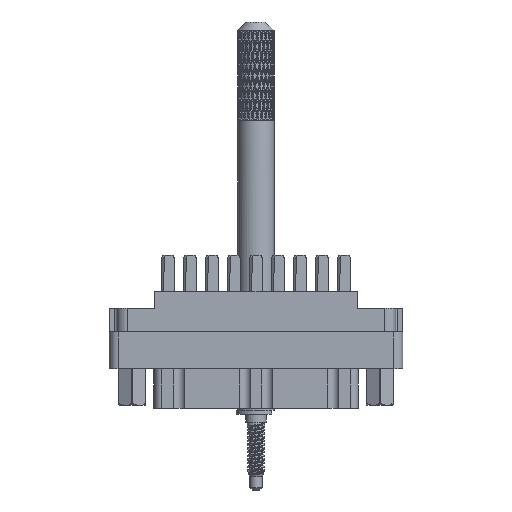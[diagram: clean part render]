
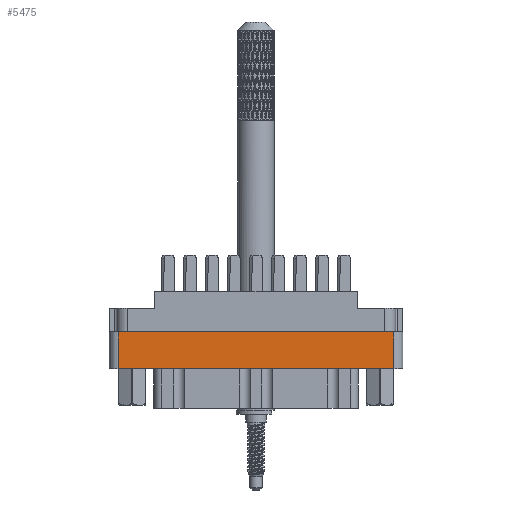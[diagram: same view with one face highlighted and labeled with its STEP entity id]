
A CAD part, front view. The second image highlights one B-rep face of the part: STEP entity #5475.
In plain terms, the highlighted planar face has unit normal (0, -1, 0).
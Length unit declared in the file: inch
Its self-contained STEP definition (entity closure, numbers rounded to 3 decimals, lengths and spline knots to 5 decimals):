
#3279 = PLANE ( 'NONE',  #110647 ) ;
#3313 = VERTEX_POINT ( 'NONE', #109894 ) ;
#5475 = ADVANCED_FACE ( 'NONE', ( #19551 ), #3279, .T. ) ;
#8591 = VECTOR ( 'NONE', #20336, 39.37008 ) ;
#11856 = LINE ( 'NONE', #29251, #79768 ) ;
#14484 = ORIENTED_EDGE ( 'NONE', *, *, #26100, .F. ) ;
#18546 = EDGE_CURVE ( 'NONE', #88867, #25865, #80310, .T. ) ;
#18998 = DIRECTION ( 'NONE',  ( 0., -1., 0. ) ) ;
#19551 = FACE_OUTER_BOUND ( 'NONE', #27443, .T. ) ;
#20336 = DIRECTION ( 'NONE',  ( 0., 0., 1. ) ) ;
#25865 = VERTEX_POINT ( 'NONE', #39438 ) ;
#26100 = EDGE_CURVE ( 'NONE', #36804, #3313, #11856, .T. ) ;
#27443 = EDGE_LOOP ( 'NONE', ( #14484, #83085, #93789, #32451 ) ) ;
#29251 = CARTESIAN_POINT ( 'NONE',  ( -0.938, -0.438, -0.798 ) ) ;
#32451 = ORIENTED_EDGE ( 'NONE', *, *, #77188, .F. ) ;
#36804 = VERTEX_POINT ( 'NONE', #90131 ) ;
#37460 = DIRECTION ( 'NONE',  ( 0., 0., -1. ) ) ;
#39438 = CARTESIAN_POINT ( 'NONE',  ( 0.938, -0.438, -0.277 ) ) ;
#44730 = VECTOR ( 'NONE', #45438, 39.37008 ) ;
#45438 = DIRECTION ( 'NONE',  ( -1., 0., 0. ) ) ;
#54375 = LINE ( 'NONE', #96449, #44730 ) ;
#55544 = EDGE_CURVE ( 'NONE', #88867, #36804, #54375, .T. ) ;
#57271 = DIRECTION ( 'NONE',  ( 1., 0., 0. ) ) ;
#77188 = EDGE_CURVE ( 'NONE', #3313, #25865, #108332, .T. ) ;
#79768 = VECTOR ( 'NONE', #105474, 39.37008 ) ;
#80310 = LINE ( 'NONE', #90946, #8591 ) ;
#83085 = ORIENTED_EDGE ( 'NONE', *, *, #55544, .F. ) ;
#88867 = VERTEX_POINT ( 'NONE', #108534 ) ;
#90131 = CARTESIAN_POINT ( 'NONE',  ( -0.938, -0.438, -0.529 ) ) ;
#90440 = CARTESIAN_POINT ( 'NONE',  ( -1., -0.438, -0.277 ) ) ;
#90946 = CARTESIAN_POINT ( 'NONE',  ( 0.938, -0.438, -0.798 ) ) ;
#93789 = ORIENTED_EDGE ( 'NONE', *, *, #18546, .T. ) ;
#96449 = CARTESIAN_POINT ( 'NONE',  ( 0.938, -0.438, -0.529 ) ) ;
#98990 = VECTOR ( 'NONE', #57271, 39.37008 ) ;
#104206 = CARTESIAN_POINT ( 'NONE',  ( -0.938, -0.438, -0.798 ) ) ;
#105474 = DIRECTION ( 'NONE',  ( 0., 0., 1. ) ) ;
#108332 = LINE ( 'NONE', #90440, #98990 ) ;
#108534 = CARTESIAN_POINT ( 'NONE',  ( 0.938, -0.438, -0.529 ) ) ;
#109894 = CARTESIAN_POINT ( 'NONE',  ( -0.938, -0.438, -0.277 ) ) ;
#110647 = AXIS2_PLACEMENT_3D ( 'NONE', #104206, #18998, #37460 ) ;
